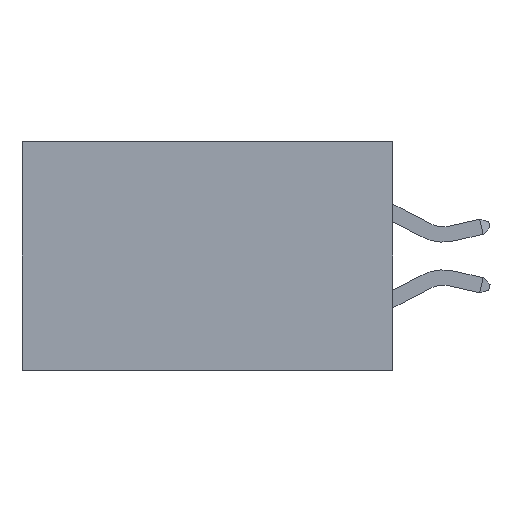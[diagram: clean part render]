
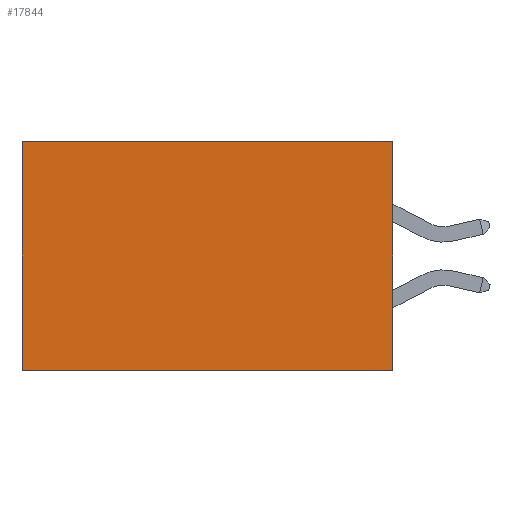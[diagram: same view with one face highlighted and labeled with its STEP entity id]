
A CAD part, left-side view. The second image highlights one B-rep face of the part: STEP entity #17844.
In plain terms, the highlighted planar face has unit normal (-1, 0, 0).
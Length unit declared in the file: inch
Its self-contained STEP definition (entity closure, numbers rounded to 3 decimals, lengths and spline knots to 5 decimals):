
#163 = CARTESIAN_POINT ( 'NONE',  ( 0.2875, 0.6, 0. ) ) ;
#911 = DIRECTION ( 'NONE',  ( 0., 0., -1. ) ) ;
#938 = EDGE_CURVE ( 'NONE', #16794, #2685, #2753, .T. ) ;
#1871 = PLANE ( 'NONE',  #2177 ) ;
#2043 = CARTESIAN_POINT ( 'NONE',  ( 0.2875, 0.6, -0.37 ) ) ;
#2177 = AXIS2_PLACEMENT_3D ( 'NONE', #3299, #4705, #14310 ) ;
#2685 = VERTEX_POINT ( 'NONE', #163 ) ;
#2753 = LINE ( 'NONE', #4874, #8882 ) ;
#3299 = CARTESIAN_POINT ( 'NONE',  ( 0.2875, 0., 0. ) ) ;
#4705 = DIRECTION ( 'NONE',  ( 1., 0., 0. ) ) ;
#4874 = CARTESIAN_POINT ( 'NONE',  ( 0.2875, 0., 0. ) ) ;
#7372 = VECTOR ( 'NONE', #911, 39.37008 ) ;
#7419 = ORIENTED_EDGE ( 'NONE', *, *, #7519, .F. ) ;
#7519 = EDGE_CURVE ( 'NONE', #16794, #14658, #8263, .T. ) ;
#8263 = LINE ( 'NONE', #12150, #7372 ) ;
#8882 = VECTOR ( 'NONE', #13574, 39.37008 ) ;
#9477 = VECTOR ( 'NONE', #17610, 39.37008 ) ;
#9797 = CARTESIAN_POINT ( 'NONE',  ( 0.2875, 0., 0. ) ) ;
#10058 = ORIENTED_EDGE ( 'NONE', *, *, #938, .T. ) ;
#12150 = CARTESIAN_POINT ( 'NONE',  ( 0.2875, 0., 0. ) ) ;
#12198 = CARTESIAN_POINT ( 'NONE',  ( 0.2875, 0., -0.37 ) ) ;
#12229 = FACE_OUTER_BOUND ( 'NONE', #12343, .T. ) ;
#12234 = CARTESIAN_POINT ( 'NONE',  ( 0.2875, 0.6, 0. ) ) ;
#12343 = EDGE_LOOP ( 'NONE', ( #12450, #17200, #7419, #10058 ) ) ;
#12362 = EDGE_CURVE ( 'NONE', #14658, #15137, #13104, .T. ) ;
#12450 = ORIENTED_EDGE ( 'NONE', *, *, #16579, .T. ) ;
#13104 = LINE ( 'NONE', #16186, #9477 ) ;
#13574 = DIRECTION ( 'NONE',  ( 0., 1., 0. ) ) ;
#14310 = DIRECTION ( 'NONE',  ( 0., 0., -1. ) ) ;
#14658 = VERTEX_POINT ( 'NONE', #12198 ) ;
#14731 = VECTOR ( 'NONE', #14874, 39.37008 ) ;
#14874 = DIRECTION ( 'NONE',  ( 0., 0., -1. ) ) ;
#15137 = VERTEX_POINT ( 'NONE', #2043 ) ;
#16186 = CARTESIAN_POINT ( 'NONE',  ( 0.2875, 0., -0.37 ) ) ;
#16579 = EDGE_CURVE ( 'NONE', #2685, #15137, #17918, .T. ) ;
#16794 = VERTEX_POINT ( 'NONE', #9797 ) ;
#17200 = ORIENTED_EDGE ( 'NONE', *, *, #12362, .F. ) ;
#17610 = DIRECTION ( 'NONE',  ( 0., 1., 0. ) ) ;
#17844 = ADVANCED_FACE ( 'NONE', ( #12229 ), #1871, .F. ) ;
#17918 = LINE ( 'NONE', #12234, #14731 ) ;
